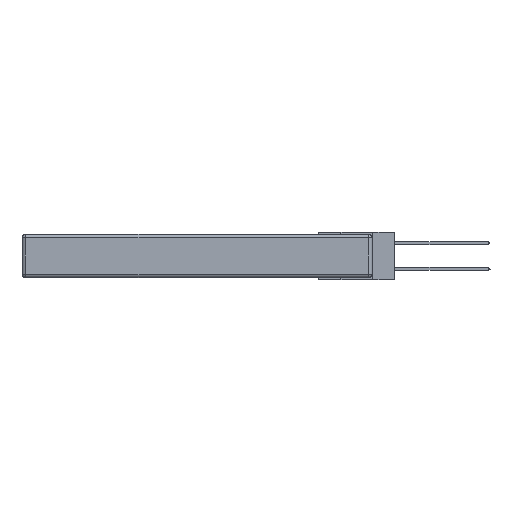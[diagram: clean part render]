
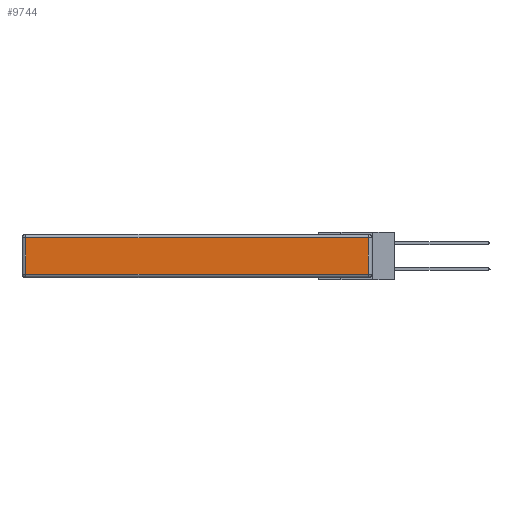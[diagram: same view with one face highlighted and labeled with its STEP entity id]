
A CAD part, left-side view. The second image highlights one B-rep face of the part: STEP entity #9744.
In plain terms, the highlighted planar face has unit normal (-1, 0, 0).
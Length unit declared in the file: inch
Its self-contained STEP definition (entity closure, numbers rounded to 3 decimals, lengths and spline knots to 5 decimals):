
#1203 = EDGE_CURVE ( 'NONE', #30186, #21264, #29171, .T. ) ;
#5051 = ORIENTED_EDGE ( 'NONE', *, *, #1203, .T. ) ;
#6613 = VECTOR ( 'NONE', #8867, 39.37008 ) ;
#8609 = CARTESIAN_POINT ( 'NONE',  ( 0., 0.03, -0.343 ) ) ;
#8615 = CARTESIAN_POINT ( 'NONE',  ( 0., 2.72, -0.03 ) ) ;
#8867 = DIRECTION ( 'NONE',  ( 0., 1., 0. ) ) ;
#9591 = CARTESIAN_POINT ( 'NONE',  ( 0., 0., -0.313 ) ) ;
#9744 = ADVANCED_FACE ( 'NONE', ( #14469 ), #14961, .T. ) ;
#10338 = LINE ( 'NONE', #29981, #6613 ) ;
#11030 = DIRECTION ( 'NONE',  ( 0., 0., 1. ) ) ;
#11805 = CARTESIAN_POINT ( 'NONE',  ( 0., 2.72, -0.313 ) ) ;
#12175 = CARTESIAN_POINT ( 'NONE',  ( 0., 2.72, -0.343 ) ) ;
#13539 = CARTESIAN_POINT ( 'NONE',  ( 0., 0.03, -0.03 ) ) ;
#14400 = DIRECTION ( 'NONE',  ( 0., -1., 0. ) ) ;
#14469 = FACE_OUTER_BOUND ( 'NONE', #30437, .T. ) ;
#14961 = PLANE ( 'NONE',  #23598 ) ;
#15610 = EDGE_CURVE ( 'NONE', #21264, #21230, #10338, .T. ) ;
#16150 = LINE ( 'NONE', #12175, #18400 ) ;
#17364 = DIRECTION ( 'NONE',  ( 0., 0., 1. ) ) ;
#17454 = VERTEX_POINT ( 'NONE', #11805 ) ;
#17672 = DIRECTION ( 'NONE',  ( 0., 0., -1. ) ) ;
#18366 = EDGE_CURVE ( 'NONE', #21230, #17454, #16150, .T. ) ;
#18400 = VECTOR ( 'NONE', #17672, 39.37008 ) ;
#19657 = ORIENTED_EDGE ( 'NONE', *, *, #20795, .T. ) ;
#20795 = EDGE_CURVE ( 'NONE', #17454, #30186, #29735, .T. ) ;
#21230 = VERTEX_POINT ( 'NONE', #8615 ) ;
#21237 = ORIENTED_EDGE ( 'NONE', *, *, #15610, .T. ) ;
#21264 = VERTEX_POINT ( 'NONE', #13539 ) ;
#21766 = DIRECTION ( 'NONE',  ( -1., 0., 0. ) ) ;
#23575 = VECTOR ( 'NONE', #11030, 39.37008 ) ;
#23598 = AXIS2_PLACEMENT_3D ( 'NONE', #24172, #21766, #17364 ) ;
#24172 = CARTESIAN_POINT ( 'NONE',  ( 0., 0., -0.343 ) ) ;
#25224 = ORIENTED_EDGE ( 'NONE', *, *, #18366, .T. ) ;
#25894 = CARTESIAN_POINT ( 'NONE',  ( 0., 0.03, -0.313 ) ) ;
#29171 = LINE ( 'NONE', #8609, #23575 ) ;
#29354 = VECTOR ( 'NONE', #14400, 39.37008 ) ;
#29735 = LINE ( 'NONE', #9591, #29354 ) ;
#29981 = CARTESIAN_POINT ( 'NONE',  ( 0., 2.75, -0.03 ) ) ;
#30186 = VERTEX_POINT ( 'NONE', #25894 ) ;
#30437 = EDGE_LOOP ( 'NONE', ( #19657, #5051, #21237, #25224 ) ) ;
